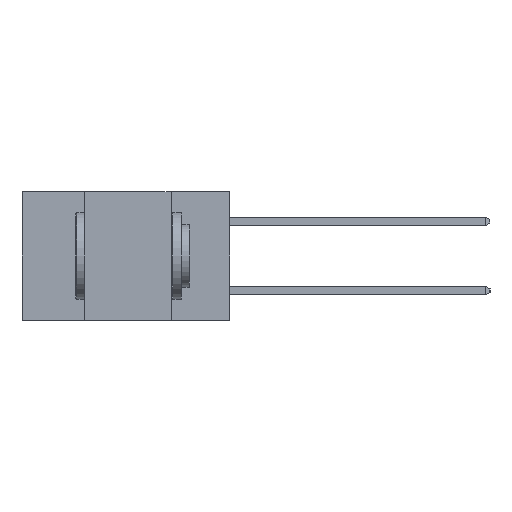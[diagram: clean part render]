
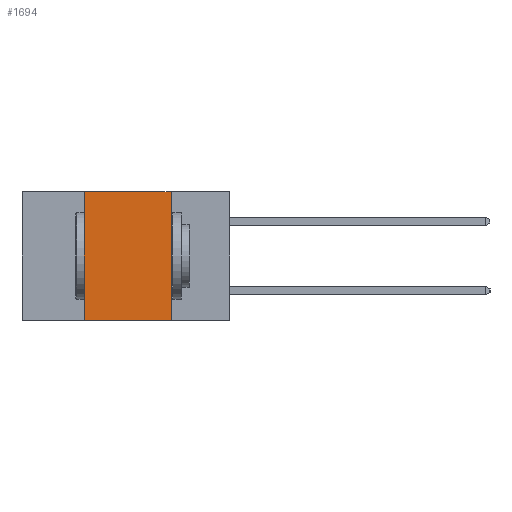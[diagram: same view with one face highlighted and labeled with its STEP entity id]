
A CAD part, left-side view. The second image highlights one B-rep face of the part: STEP entity #1694.
In plain terms, the highlighted planar face has unit normal (-1, 0, 0).
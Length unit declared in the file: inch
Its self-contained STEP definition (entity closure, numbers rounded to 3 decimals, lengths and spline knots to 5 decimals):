
#1287 = CARTESIAN_POINT ( 'NONE',  ( 0., 0.6, 0. ) ) ;
#1429 = DIRECTION ( 'NONE',  ( 0., -1., 0. ) ) ;
#1694 = ADVANCED_FACE ( 'NONE', ( #8865 ), #10129, .F. ) ;
#1917 = VERTEX_POINT ( 'NONE', #3509 ) ;
#2001 = VECTOR ( 'NONE', #2076, 39.37008 ) ;
#2076 = DIRECTION ( 'NONE',  ( 0., -1., 0. ) ) ;
#2225 = CARTESIAN_POINT ( 'NONE',  ( 0., 0.6, -0.37 ) ) ;
#2229 = VERTEX_POINT ( 'NONE', #9408 ) ;
#2262 = LINE ( 'NONE', #1287, #2001 ) ;
#2989 = EDGE_CURVE ( 'NONE', #1917, #8154, #5608, .T. ) ;
#3509 = CARTESIAN_POINT ( 'NONE',  ( 0., 0.17, 0. ) ) ;
#4155 = EDGE_LOOP ( 'NONE', ( #5790, #9608, #4557, #9356 ) ) ;
#4281 = EDGE_CURVE ( 'NONE', #2229, #5855, #7770, .T. ) ;
#4472 = CARTESIAN_POINT ( 'NONE',  ( 0., 0.42, 0. ) ) ;
#4557 = ORIENTED_EDGE ( 'NONE', *, *, #4281, .F. ) ;
#5009 = CARTESIAN_POINT ( 'NONE',  ( 0., 0.17, -0.37 ) ) ;
#5371 = CARTESIAN_POINT ( 'NONE',  ( 0., 0.42, -0.37 ) ) ;
#5447 = DIRECTION ( 'NONE',  ( 0., 0., 1. ) ) ;
#5608 = LINE ( 'NONE', #9425, #7030 ) ;
#5790 = ORIENTED_EDGE ( 'NONE', *, *, #2989, .F. ) ;
#5812 = EDGE_CURVE ( 'NONE', #5855, #1917, #2262, .T. ) ;
#5855 = VERTEX_POINT ( 'NONE', #4472 ) ;
#7030 = VECTOR ( 'NONE', #9671, 39.37008 ) ;
#7053 = VECTOR ( 'NONE', #1429, 39.37008 ) ;
#7732 = EDGE_CURVE ( 'NONE', #2229, #8154, #9200, .T. ) ;
#7770 = LINE ( 'NONE', #5371, #9658 ) ;
#7800 = DIRECTION ( 'NONE',  ( 0., 0., -1. ) ) ;
#8154 = VERTEX_POINT ( 'NONE', #5009 ) ;
#8865 = FACE_OUTER_BOUND ( 'NONE', #4155, .T. ) ;
#9200 = LINE ( 'NONE', #2225, #7053 ) ;
#9356 = ORIENTED_EDGE ( 'NONE', *, *, #7732, .T. ) ;
#9408 = CARTESIAN_POINT ( 'NONE',  ( 0., 0.42, -0.37 ) ) ;
#9425 = CARTESIAN_POINT ( 'NONE',  ( 0., 0.17, -0.37 ) ) ;
#9608 = ORIENTED_EDGE ( 'NONE', *, *, #5812, .F. ) ;
#9658 = VECTOR ( 'NONE', #5447, 39.37008 ) ;
#9671 = DIRECTION ( 'NONE',  ( 0., 0., -1. ) ) ;
#10072 = CARTESIAN_POINT ( 'NONE',  ( 0., 0.6, 0. ) ) ;
#10092 = DIRECTION ( 'NONE',  ( 1., 0., 0. ) ) ;
#10129 = PLANE ( 'NONE',  #10189 ) ;
#10189 = AXIS2_PLACEMENT_3D ( 'NONE', #10072, #10092, #7800 ) ;
